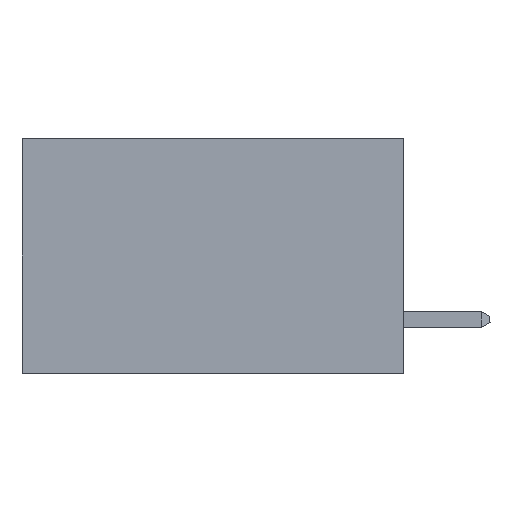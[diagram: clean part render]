
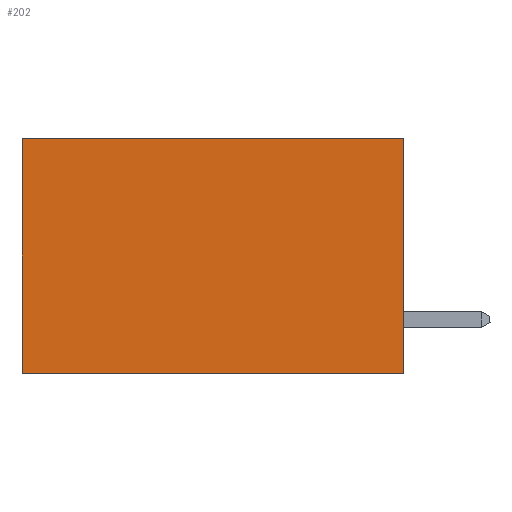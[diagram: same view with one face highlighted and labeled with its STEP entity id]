
A CAD part, left-side view. The second image highlights one B-rep face of the part: STEP entity #202.
In plain terms, the highlighted planar face has unit normal (-1, 0, 0).
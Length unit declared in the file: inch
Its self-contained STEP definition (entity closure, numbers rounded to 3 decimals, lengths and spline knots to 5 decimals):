
#202 = ADVANCED_FACE ( 'NONE', ( #17777 ), #14779, .F. ) ;
#1361 = EDGE_CURVE ( 'NONE', #23145, #22957, #1770, .T. ) ;
#1432 = CARTESIAN_POINT ( 'NONE',  ( 0.2875, 0., 0. ) ) ;
#1668 = VECTOR ( 'NONE', #22699, 39.37008 ) ;
#1770 = LINE ( 'NONE', #6923, #6783 ) ;
#2809 = CARTESIAN_POINT ( 'NONE',  ( 0.2875, 0., 0. ) ) ;
#2933 = LINE ( 'NONE', #11417, #23504 ) ;
#4050 = EDGE_CURVE ( 'NONE', #23145, #15598, #19014, .T. ) ;
#4696 = DIRECTION ( 'NONE',  ( 0., 1., 0. ) ) ;
#5911 = VERTEX_POINT ( 'NONE', #20654 ) ;
#5944 = ORIENTED_EDGE ( 'NONE', *, *, #4050, .F. ) ;
#6742 = CARTESIAN_POINT ( 'NONE',  ( 0.2875, 0.6, 0. ) ) ;
#6783 = VECTOR ( 'NONE', #4696, 39.37008 ) ;
#6923 = CARTESIAN_POINT ( 'NONE',  ( 0.2875, 0., 0. ) ) ;
#7490 = DIRECTION ( 'NONE',  ( 0., 0., -1. ) ) ;
#8513 = CARTESIAN_POINT ( 'NONE',  ( 0.2875, 0.6, 0. ) ) ;
#9501 = DIRECTION ( 'NONE',  ( 0., 1., 0. ) ) ;
#10302 = EDGE_LOOP ( 'NONE', ( #17959, #16920, #5944, #23109 ) ) ;
#11417 = CARTESIAN_POINT ( 'NONE',  ( 0.2875, 0., -0.37 ) ) ;
#11504 = EDGE_CURVE ( 'NONE', #15598, #5911, #2933, .T. ) ;
#14191 = LINE ( 'NONE', #6742, #1668 ) ;
#14779 = PLANE ( 'NONE',  #17401 ) ;
#14877 = CARTESIAN_POINT ( 'NONE',  ( 0.2875, 0., 0. ) ) ;
#15598 = VERTEX_POINT ( 'NONE', #21606 ) ;
#16585 = EDGE_CURVE ( 'NONE', #22957, #5911, #14191, .T. ) ;
#16920 = ORIENTED_EDGE ( 'NONE', *, *, #11504, .F. ) ;
#17401 = AXIS2_PLACEMENT_3D ( 'NONE', #2809, #22767, #7490 ) ;
#17777 = FACE_OUTER_BOUND ( 'NONE', #10302, .T. ) ;
#17959 = ORIENTED_EDGE ( 'NONE', *, *, #16585, .T. ) ;
#18393 = VECTOR ( 'NONE', #19062, 39.37008 ) ;
#19014 = LINE ( 'NONE', #14877, #18393 ) ;
#19062 = DIRECTION ( 'NONE',  ( 0., 0., -1. ) ) ;
#20654 = CARTESIAN_POINT ( 'NONE',  ( 0.2875, 0.6, -0.37 ) ) ;
#21606 = CARTESIAN_POINT ( 'NONE',  ( 0.2875, 0., -0.37 ) ) ;
#22699 = DIRECTION ( 'NONE',  ( 0., 0., -1. ) ) ;
#22767 = DIRECTION ( 'NONE',  ( 1., 0., 0. ) ) ;
#22957 = VERTEX_POINT ( 'NONE', #8513 ) ;
#23109 = ORIENTED_EDGE ( 'NONE', *, *, #1361, .T. ) ;
#23145 = VERTEX_POINT ( 'NONE', #1432 ) ;
#23504 = VECTOR ( 'NONE', #9501, 39.37008 ) ;
